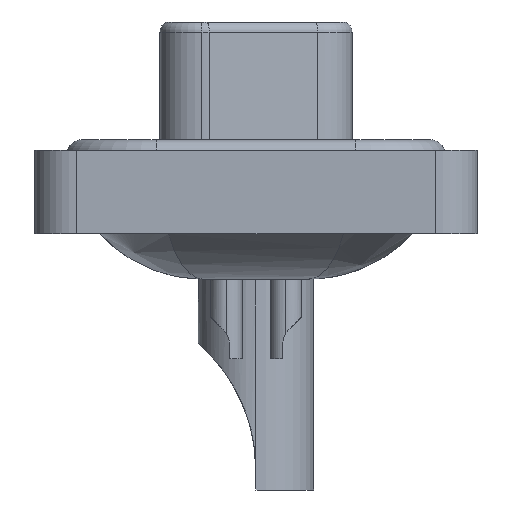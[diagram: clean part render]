
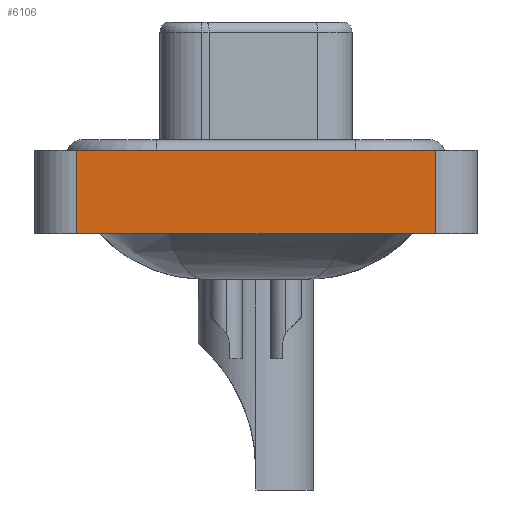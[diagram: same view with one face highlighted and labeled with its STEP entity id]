
A CAD part, left-side view. The second image highlights one B-rep face of the part: STEP entity #6106.
In plain terms, the highlighted planar face has unit normal (-1, 0, 0).
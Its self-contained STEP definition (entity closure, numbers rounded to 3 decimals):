
#580 = LINE ( 'NONE', #5211, #1044 ) ;
#643 = VECTOR ( 'NONE', #2053, 1000. ) ;
#1044 = VECTOR ( 'NONE', #15406, 1000. ) ;
#1337 = VECTOR ( 'NONE', #19444, 1000. ) ;
#1366 = DIRECTION ( 'NONE',  ( -1., 0., 0. ) ) ;
#2053 = DIRECTION ( 'NONE',  ( 0., 0., 1. ) ) ;
#2170 = ORIENTED_EDGE ( 'NONE', *, *, #13041, .T. ) ;
#2259 = ORIENTED_EDGE ( 'NONE', *, *, #13181, .F. ) ;
#5211 = CARTESIAN_POINT ( 'NONE',  ( -7.3, -8.55, 0.4 ) ) ;
#6106 = ADVANCED_FACE ( 'NONE', ( #19189 ), #10928, .T. ) ;
#6832 = VECTOR ( 'NONE', #15039, 1000. ) ;
#7091 = ORIENTED_EDGE ( 'NONE', *, *, #13404, .T. ) ;
#7125 = VERTEX_POINT ( 'NONE', #7177 ) ;
#7177 = CARTESIAN_POINT ( 'NONE',  ( -7.3, 8.55, -3.6 ) ) ;
#7618 = CARTESIAN_POINT ( 'NONE',  ( -7.3, -8.55, -3.6 ) ) ;
#7735 = AXIS2_PLACEMENT_3D ( 'NONE', #11033, #1366, #14245 ) ;
#8888 = VERTEX_POINT ( 'NONE', #15210 ) ;
#9692 = EDGE_LOOP ( 'NONE', ( #2170, #11013, #2259, #7091 ) ) ;
#10136 = VERTEX_POINT ( 'NONE', #7618 ) ;
#10928 = PLANE ( 'NONE',  #7735 ) ;
#11013 = ORIENTED_EDGE ( 'NONE', *, *, #14498, .F. ) ;
#11033 = CARTESIAN_POINT ( 'NONE',  ( -7.3, -8.55, -3.6 ) ) ;
#11809 = LINE ( 'NONE', #19773, #6832 ) ;
#12482 = CARTESIAN_POINT ( 'NONE',  ( -7.3, 8.55, 0.4 ) ) ;
#12566 = LINE ( 'NONE', #17837, #1337 ) ;
#13041 = EDGE_CURVE ( 'NONE', #10136, #8888, #16756, .T. ) ;
#13181 = EDGE_CURVE ( 'NONE', #7125, #21119, #12566, .T. ) ;
#13404 = EDGE_CURVE ( 'NONE', #7125, #10136, #11809, .T. ) ;
#14245 = DIRECTION ( 'NONE',  ( 0., 0., 1. ) ) ;
#14451 = CARTESIAN_POINT ( 'NONE',  ( -7.3, -8.55, -3.6 ) ) ;
#14498 = EDGE_CURVE ( 'NONE', #21119, #8888, #580, .T. ) ;
#15039 = DIRECTION ( 'NONE',  ( 0., -1., 0. ) ) ;
#15210 = CARTESIAN_POINT ( 'NONE',  ( -7.3, -8.55, 0.4 ) ) ;
#15406 = DIRECTION ( 'NONE',  ( 0., -1., 0. ) ) ;
#16756 = LINE ( 'NONE', #14451, #643 ) ;
#17837 = CARTESIAN_POINT ( 'NONE',  ( -7.3, 8.55, -3.6 ) ) ;
#19189 = FACE_OUTER_BOUND ( 'NONE', #9692, .T. ) ;
#19444 = DIRECTION ( 'NONE',  ( 0., 0., 1. ) ) ;
#19773 = CARTESIAN_POINT ( 'NONE',  ( -7.3, -8.55, -3.6 ) ) ;
#21119 = VERTEX_POINT ( 'NONE', #12482 ) ;
